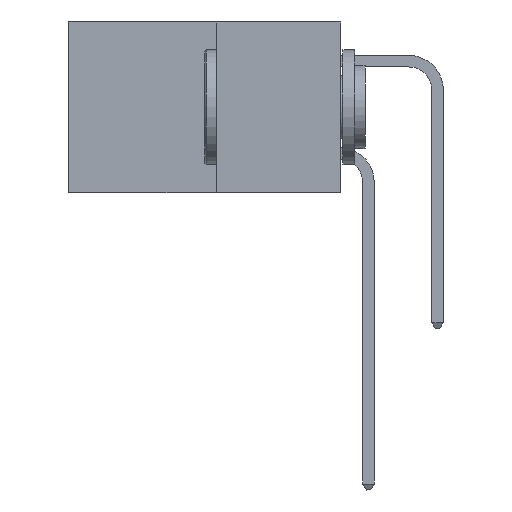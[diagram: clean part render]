
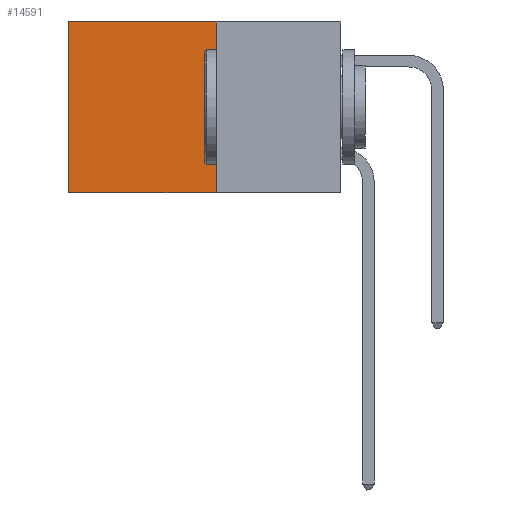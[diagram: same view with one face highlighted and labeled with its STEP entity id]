
A CAD part, left-side view. The second image highlights one B-rep face of the part: STEP entity #14591.
In plain terms, the highlighted planar face has unit normal (-1, 0, 0).
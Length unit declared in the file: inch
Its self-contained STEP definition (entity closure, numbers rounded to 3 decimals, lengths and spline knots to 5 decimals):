
#195 = EDGE_CURVE ( 'NONE', #3484, #26461, #3471, .T. ) ;
#2872 = VECTOR ( 'NONE', #14440, 39.37008 ) ;
#3471 = LINE ( 'NONE', #4163, #14617 ) ;
#3484 = VERTEX_POINT ( 'NONE', #10275 ) ;
#4163 = CARTESIAN_POINT ( 'NONE',  ( 0.277, 0.59, -0.37 ) ) ;
#4828 = EDGE_CURVE ( 'NONE', #19783, #26461, #20764, .T. ) ;
#5184 = EDGE_CURVE ( 'NONE', #24256, #3484, #15962, .T. ) ;
#6781 = CARTESIAN_POINT ( 'NONE',  ( 0.277, 0.27, -0.37 ) ) ;
#8721 = VECTOR ( 'NONE', #22161, 39.37008 ) ;
#9824 = CARTESIAN_POINT ( 'NONE',  ( 0.277, 0.27, -0.37 ) ) ;
#10275 = CARTESIAN_POINT ( 'NONE',  ( 0.277, 0.59, 0. ) ) ;
#11090 = VECTOR ( 'NONE', #26139, 39.37008 ) ;
#11249 = DIRECTION ( 'NONE',  ( 0., 0., -1. ) ) ;
#13051 = DIRECTION ( 'NONE',  ( 0., 0., -1. ) ) ;
#13782 = EDGE_CURVE ( 'NONE', #24256, #19783, #14928, .T. ) ;
#14408 = AXIS2_PLACEMENT_3D ( 'NONE', #6781, #25258, #13051 ) ;
#14440 = DIRECTION ( 'NONE',  ( 0., 1., 0. ) ) ;
#14591 = ADVANCED_FACE ( 'NONE', ( #18706 ), #19151, .F. ) ;
#14617 = VECTOR ( 'NONE', #11249, 39.37008 ) ;
#14621 = CARTESIAN_POINT ( 'NONE',  ( 0.277, 0.27, -0.37 ) ) ;
#14928 = LINE ( 'NONE', #9824, #8721 ) ;
#15962 = LINE ( 'NONE', #26165, #11090 ) ;
#18706 = FACE_OUTER_BOUND ( 'NONE', #26262, .T. ) ;
#19151 = PLANE ( 'NONE',  #14408 ) ;
#19783 = VERTEX_POINT ( 'NONE', #21552 ) ;
#20764 = LINE ( 'NONE', #14621, #2872 ) ;
#21552 = CARTESIAN_POINT ( 'NONE',  ( 0.277, 0.27, -0.37 ) ) ;
#21755 = CARTESIAN_POINT ( 'NONE',  ( 0.277, 0.27, 0. ) ) ;
#21840 = ORIENTED_EDGE ( 'NONE', *, *, #5184, .T. ) ;
#22031 = ORIENTED_EDGE ( 'NONE', *, *, #13782, .F. ) ;
#22161 = DIRECTION ( 'NONE',  ( 0., 0., -1. ) ) ;
#22182 = ORIENTED_EDGE ( 'NONE', *, *, #4828, .F. ) ;
#22271 = ORIENTED_EDGE ( 'NONE', *, *, #195, .T. ) ;
#24256 = VERTEX_POINT ( 'NONE', #21755 ) ;
#25070 = CARTESIAN_POINT ( 'NONE',  ( 0.277, 0.59, -0.37 ) ) ;
#25258 = DIRECTION ( 'NONE',  ( 1., 0., 0. ) ) ;
#26139 = DIRECTION ( 'NONE',  ( 0., 1., 0. ) ) ;
#26165 = CARTESIAN_POINT ( 'NONE',  ( 0.277, 0.27, 0. ) ) ;
#26262 = EDGE_LOOP ( 'NONE', ( #22271, #22182, #22031, #21840 ) ) ;
#26461 = VERTEX_POINT ( 'NONE', #25070 ) ;
